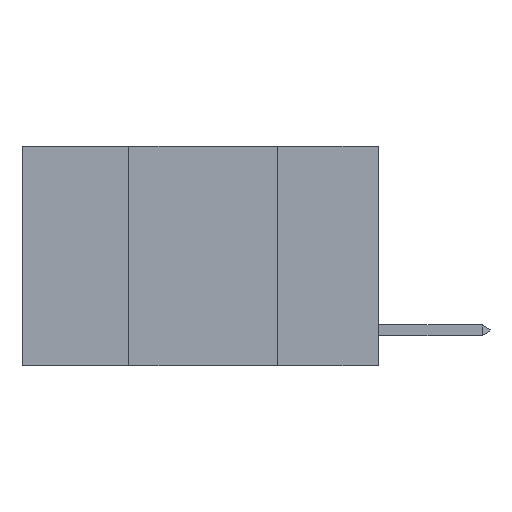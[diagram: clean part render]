
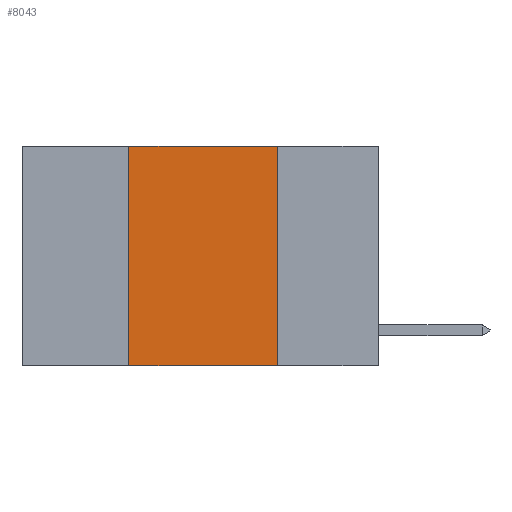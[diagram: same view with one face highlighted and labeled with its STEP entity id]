
A CAD part, left-side view. The second image highlights one B-rep face of the part: STEP entity #8043.
In plain terms, the highlighted planar face has unit normal (-1, 0, 0).
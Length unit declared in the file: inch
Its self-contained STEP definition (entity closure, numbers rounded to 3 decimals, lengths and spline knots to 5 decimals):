
#115 = EDGE_CURVE ( 'NONE', #940, #7759, #4393, .T. ) ;
#578 = DIRECTION ( 'NONE',  ( 0., 0., -1. ) ) ;
#724 = LINE ( 'NONE', #14198, #9412 ) ;
#838 = DIRECTION ( 'NONE',  ( 0., 0., 1. ) ) ;
#897 = CARTESIAN_POINT ( 'NONE',  ( 0., 0.6, 0. ) ) ;
#940 = VERTEX_POINT ( 'NONE', #2525 ) ;
#1348 = VERTEX_POINT ( 'NONE', #13402 ) ;
#1479 = CARTESIAN_POINT ( 'NONE',  ( 0., 0.42, 0. ) ) ;
#2068 = VECTOR ( 'NONE', #838, 39.37008 ) ;
#2525 = CARTESIAN_POINT ( 'NONE',  ( 0., 0.17, 0. ) ) ;
#3632 = ORIENTED_EDGE ( 'NONE', *, *, #10860, .F. ) ;
#3942 = LINE ( 'NONE', #11097, #4712 ) ;
#4393 = LINE ( 'NONE', #9352, #4838 ) ;
#4712 = VECTOR ( 'NONE', #8911, 39.37008 ) ;
#4838 = VECTOR ( 'NONE', #578, 39.37008 ) ;
#5380 = VERTEX_POINT ( 'NONE', #1479 ) ;
#6367 = EDGE_CURVE ( 'NONE', #1348, #5380, #14458, .T. ) ;
#6589 = CARTESIAN_POINT ( 'NONE',  ( 0., 0.17, -0.37 ) ) ;
#7759 = VERTEX_POINT ( 'NONE', #6589 ) ;
#8043 = ADVANCED_FACE ( 'NONE', ( #14517 ), #8454, .F. ) ;
#8454 = PLANE ( 'NONE',  #13767 ) ;
#8638 = EDGE_CURVE ( 'NONE', #1348, #7759, #3942, .T. ) ;
#8911 = DIRECTION ( 'NONE',  ( 0., -1., 0. ) ) ;
#9352 = CARTESIAN_POINT ( 'NONE',  ( 0., 0.17, 0. ) ) ;
#9412 = VECTOR ( 'NONE', #15505, 39.37008 ) ;
#10285 = ORIENTED_EDGE ( 'NONE', *, *, #8638, .T. ) ;
#10860 = EDGE_CURVE ( 'NONE', #5380, #940, #724, .T. ) ;
#10956 = DIRECTION ( 'NONE',  ( 0., 0., -1. ) ) ;
#11052 = CARTESIAN_POINT ( 'NONE',  ( 0., 0.42, 0. ) ) ;
#11097 = CARTESIAN_POINT ( 'NONE',  ( 0., 0.6, -0.37 ) ) ;
#11243 = ORIENTED_EDGE ( 'NONE', *, *, #115, .F. ) ;
#13241 = DIRECTION ( 'NONE',  ( 1., 0., 0. ) ) ;
#13402 = CARTESIAN_POINT ( 'NONE',  ( 0., 0.42, -0.37 ) ) ;
#13767 = AXIS2_PLACEMENT_3D ( 'NONE', #897, #13241, #10956 ) ;
#14198 = CARTESIAN_POINT ( 'NONE',  ( 0., 0.6, 0. ) ) ;
#14458 = LINE ( 'NONE', #11052, #2068 ) ;
#14517 = FACE_OUTER_BOUND ( 'NONE', #15114, .T. ) ;
#15114 = EDGE_LOOP ( 'NONE', ( #11243, #3632, #15643, #10285 ) ) ;
#15505 = DIRECTION ( 'NONE',  ( 0., -1., 0. ) ) ;
#15643 = ORIENTED_EDGE ( 'NONE', *, *, #6367, .F. ) ;
